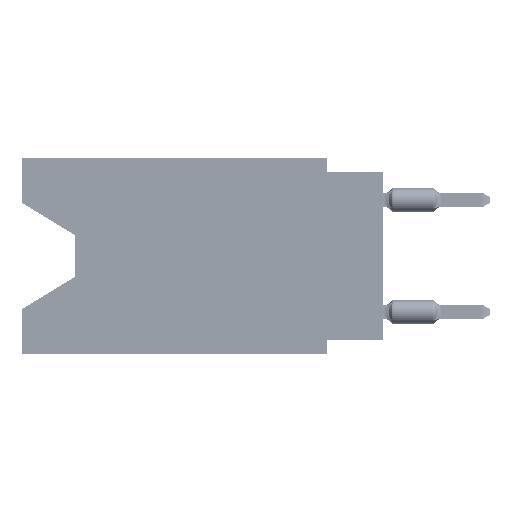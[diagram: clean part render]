
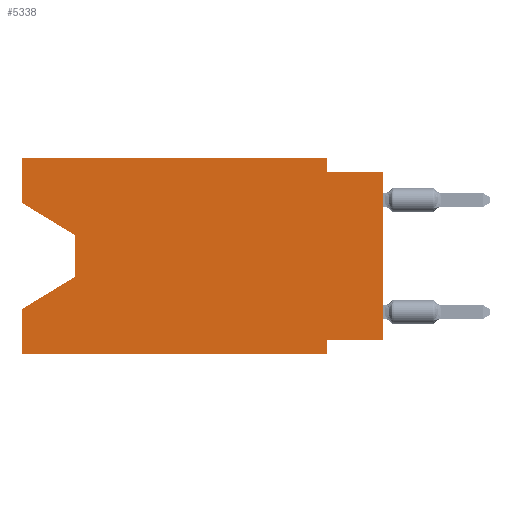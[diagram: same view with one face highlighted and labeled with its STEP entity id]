
A CAD part, left-side view. The second image highlights one B-rep face of the part: STEP entity #5338.
In plain terms, the highlighted planar face has unit normal (-1, 0, 0).
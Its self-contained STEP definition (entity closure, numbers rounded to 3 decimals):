
#735 = CARTESIAN_POINT ( 'NONE',  ( 0., 16.383, 0. ) ) ;
#2081 = CARTESIAN_POINT ( 'NONE',  ( 0., 16.383, -6.852 ) ) ;
#2373 = DIRECTION ( 'NONE',  ( 0., 0., 1. ) ) ;
#2766 = ORIENTED_EDGE ( 'NONE', *, *, #31526, .T. ) ;
#3571 = CARTESIAN_POINT ( 'NONE',  ( 0., 2.54, -8.89 ) ) ;
#4767 = CARTESIAN_POINT ( 'NONE',  ( 0., 2.54, 0. ) ) ;
#4783 = VERTEX_POINT ( 'NONE', #64614 ) ;
#5338 = ADVANCED_FACE ( 'NONE', ( #23233 ), #81678, .F. ) ;
#6061 = LINE ( 'NONE', #13931, #84470 ) ;
#6349 = DIRECTION ( 'NONE',  ( 0., 1., 0. ) ) ;
#6916 = DIRECTION ( 'NONE',  ( 0., -1., 0. ) ) ;
#7055 = DIRECTION ( 'NONE',  ( 1., 0., 0. ) ) ;
#7515 = EDGE_CURVE ( 'NONE', #22755, #62136, #51004, .T. ) ;
#8056 = EDGE_CURVE ( 'NONE', #86875, #84373, #48661, .T. ) ;
#11912 = ORIENTED_EDGE ( 'NONE', *, *, #41970, .F. ) ;
#12776 = VECTOR ( 'NONE', #74684, 1000. ) ;
#13352 = ORIENTED_EDGE ( 'NONE', *, *, #74847, .T. ) ;
#13931 = CARTESIAN_POINT ( 'NONE',  ( 0., 16.383, 0. ) ) ;
#14018 = ORIENTED_EDGE ( 'NONE', *, *, #7515, .F. ) ;
#14435 = CARTESIAN_POINT ( 'NONE',  ( 0., 16.383, 0. ) ) ;
#15131 = LINE ( 'NONE', #75979, #90978 ) ;
#15684 = AXIS2_PLACEMENT_3D ( 'NONE', #14435, #7055, #53155 ) ;
#18834 = ORIENTED_EDGE ( 'NONE', *, *, #41077, .F. ) ;
#22755 = VERTEX_POINT ( 'NONE', #92926 ) ;
#23127 = CARTESIAN_POINT ( 'NONE',  ( 0., 2.54, 0. ) ) ;
#23233 = FACE_OUTER_BOUND ( 'NONE', #86429, .T. ) ;
#23328 = ORIENTED_EDGE ( 'NONE', *, *, #36016, .T. ) ;
#26380 = LINE ( 'NONE', #39673, #43002 ) ;
#26551 = LINE ( 'NONE', #28474, #75910 ) ;
#27225 = VERTEX_POINT ( 'NONE', #3571 ) ;
#27508 = DIRECTION ( 'NONE',  ( 0., -0.855, -0.519 ) ) ;
#27995 = VECTOR ( 'NONE', #88209, 1000. ) ;
#28050 = ORIENTED_EDGE ( 'NONE', *, *, #30013, .F. ) ;
#28474 = CARTESIAN_POINT ( 'NONE',  ( 0., 16.383, -8.89 ) ) ;
#30013 = EDGE_CURVE ( 'NONE', #30891, #37097, #6061, .T. ) ;
#30891 = VERTEX_POINT ( 'NONE', #71157 ) ;
#31344 = VERTEX_POINT ( 'NONE', #61072 ) ;
#31526 = EDGE_CURVE ( 'NONE', #4783, #37097, #15131, .T. ) ;
#31661 = VECTOR ( 'NONE', #67463, 1000. ) ;
#34209 = LINE ( 'NONE', #4767, #27995 ) ;
#35821 = LINE ( 'NONE', #94773, #36030 ) ;
#36016 = EDGE_CURVE ( 'NONE', #30891, #27225, #26551, .T. ) ;
#36030 = VECTOR ( 'NONE', #27508, 1000. ) ;
#36334 = ORIENTED_EDGE ( 'NONE', *, *, #57744, .T. ) ;
#37097 = VERTEX_POINT ( 'NONE', #2081 ) ;
#39673 = CARTESIAN_POINT ( 'NONE',  ( 0., 0., 0. ) ) ;
#40725 = CARTESIAN_POINT ( 'NONE',  ( 0., 16.383, 0. ) ) ;
#41077 = EDGE_CURVE ( 'NONE', #31344, #92150, #53704, .T. ) ;
#41970 = EDGE_CURVE ( 'NONE', #62136, #27225, #46105, .T. ) ;
#43002 = VECTOR ( 'NONE', #2373, 1000. ) ;
#43627 = CARTESIAN_POINT ( 'NONE',  ( 0., 0., -8.255 ) ) ;
#44712 = LINE ( 'NONE', #95798, #12776 ) ;
#46105 = LINE ( 'NONE', #83449, #93009 ) ;
#47271 = CARTESIAN_POINT ( 'NONE',  ( 0., 13.97, -3.505 ) ) ;
#48661 = LINE ( 'NONE', #78652, #77272 ) ;
#49432 = EDGE_CURVE ( 'NONE', #60353, #86875, #34209, .T. ) ;
#51004 = LINE ( 'NONE', #43627, #92814 ) ;
#52783 = ORIENTED_EDGE ( 'NONE', *, *, #8056, .F. ) ;
#53155 = DIRECTION ( 'NONE',  ( 0., 0., -1. ) ) ;
#53704 = LINE ( 'NONE', #76311, #72451 ) ;
#57744 = EDGE_CURVE ( 'NONE', #31344, #75871, #35821, .T. ) ;
#58562 = DIRECTION ( 'NONE',  ( 0., 0., 1. ) ) ;
#60353 = VERTEX_POINT ( 'NONE', #23127 ) ;
#61006 = EDGE_CURVE ( 'NONE', #22755, #84373, #26380, .T. ) ;
#61072 = CARTESIAN_POINT ( 'NONE',  ( 0., 16.383, -2.038 ) ) ;
#62136 = VERTEX_POINT ( 'NONE', #63226 ) ;
#62621 = ORIENTED_EDGE ( 'NONE', *, *, #61006, .T. ) ;
#63226 = CARTESIAN_POINT ( 'NONE',  ( 0., 2.54, -8.255 ) ) ;
#64614 = CARTESIAN_POINT ( 'NONE',  ( 0., 13.97, -5.385 ) ) ;
#65700 = CARTESIAN_POINT ( 'NONE',  ( 0., 0., -0.635 ) ) ;
#66973 = LINE ( 'NONE', #735, #31661 ) ;
#67463 = DIRECTION ( 'NONE',  ( 0., -1., 0. ) ) ;
#69055 = DIRECTION ( 'NONE',  ( 0., 0.855, -0.519 ) ) ;
#71156 = EDGE_CURVE ( 'NONE', #92150, #60353, #66973, .T. ) ;
#71157 = CARTESIAN_POINT ( 'NONE',  ( 0., 16.383, -8.89 ) ) ;
#72451 = VECTOR ( 'NONE', #91523, 1000. ) ;
#74684 = DIRECTION ( 'NONE',  ( 0., 0., -1. ) ) ;
#74847 = EDGE_CURVE ( 'NONE', #75871, #4783, #44712, .T. ) ;
#75871 = VERTEX_POINT ( 'NONE', #47271 ) ;
#75910 = VECTOR ( 'NONE', #94781, 1000. ) ;
#75979 = CARTESIAN_POINT ( 'NONE',  ( 0., 13.97, -5.385 ) ) ;
#76083 = DIRECTION ( 'NONE',  ( 0., 0., -1. ) ) ;
#76311 = CARTESIAN_POINT ( 'NONE',  ( 0., 16.383, 0. ) ) ;
#77131 = CARTESIAN_POINT ( 'NONE',  ( 0., 2.54, -0.635 ) ) ;
#77272 = VECTOR ( 'NONE', #6916, 1000. ) ;
#78652 = CARTESIAN_POINT ( 'NONE',  ( 0., 0., -0.635 ) ) ;
#81678 = PLANE ( 'NONE',  #15684 ) ;
#83449 = CARTESIAN_POINT ( 'NONE',  ( 0., 2.54, -8.89 ) ) ;
#84373 = VERTEX_POINT ( 'NONE', #65700 ) ;
#84470 = VECTOR ( 'NONE', #58562, 1000. ) ;
#86429 = EDGE_LOOP ( 'NONE', ( #36334, #13352, #2766, #28050, #23328, #11912, #14018, #62621, #52783, #90096, #86524, #18834 ) ) ;
#86524 = ORIENTED_EDGE ( 'NONE', *, *, #71156, .F. ) ;
#86875 = VERTEX_POINT ( 'NONE', #77131 ) ;
#88209 = DIRECTION ( 'NONE',  ( 0., 0., -1. ) ) ;
#90096 = ORIENTED_EDGE ( 'NONE', *, *, #49432, .F. ) ;
#90978 = VECTOR ( 'NONE', #69055, 1000. ) ;
#91523 = DIRECTION ( 'NONE',  ( 0., 0., 1. ) ) ;
#92150 = VERTEX_POINT ( 'NONE', #40725 ) ;
#92814 = VECTOR ( 'NONE', #6349, 1000. ) ;
#92926 = CARTESIAN_POINT ( 'NONE',  ( 0., 0., -8.255 ) ) ;
#93009 = VECTOR ( 'NONE', #76083, 1000. ) ;
#94773 = CARTESIAN_POINT ( 'NONE',  ( 0., 16.383, -2.038 ) ) ;
#94781 = DIRECTION ( 'NONE',  ( 0., -1., 0. ) ) ;
#95798 = CARTESIAN_POINT ( 'NONE',  ( 0., 13.97, -3.505 ) ) ;
